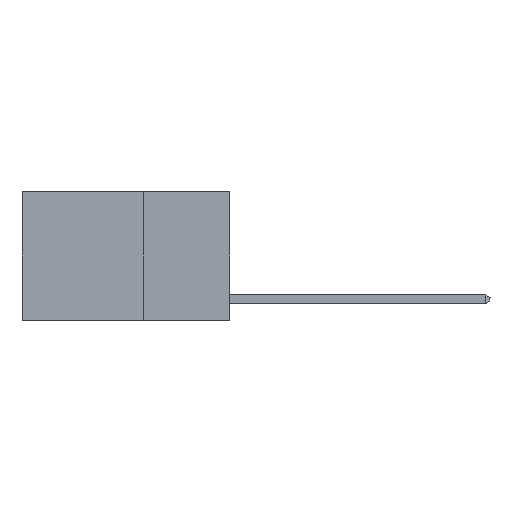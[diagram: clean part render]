
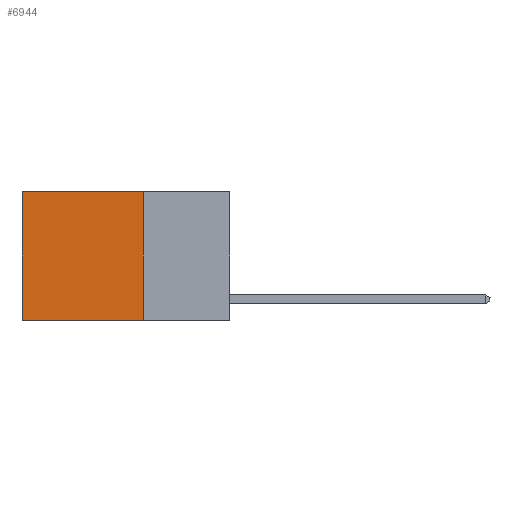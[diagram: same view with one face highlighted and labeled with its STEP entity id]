
A CAD part, left-side view. The second image highlights one B-rep face of the part: STEP entity #6944.
In plain terms, the highlighted planar face has unit normal (-1, 0, 0).
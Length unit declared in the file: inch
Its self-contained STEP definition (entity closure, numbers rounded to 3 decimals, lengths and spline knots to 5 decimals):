
#1511 = CARTESIAN_POINT ( 'NONE',  ( 0.2625, 0.6, 0. ) ) ;
#2261 = DIRECTION ( 'NONE',  ( 0., 1., 0. ) ) ;
#2919 = VERTEX_POINT ( 'NONE', #18319 ) ;
#5764 = FACE_OUTER_BOUND ( 'NONE', #28611, .T. ) ;
#5936 = DIRECTION ( 'NONE',  ( 0., 0., -1. ) ) ;
#6759 = CARTESIAN_POINT ( 'NONE',  ( 0.2625, 0.6, -0.37 ) ) ;
#6944 = ADVANCED_FACE ( 'NONE', ( #5764 ), #14652, .F. ) ;
#8259 = EDGE_CURVE ( 'NONE', #2919, #14107, #26554, .T. ) ;
#9072 = VECTOR ( 'NONE', #15475, 39.37008 ) ;
#10255 = CARTESIAN_POINT ( 'NONE',  ( 0.2625, 0.25, 0. ) ) ;
#11265 = DIRECTION ( 'NONE',  ( 0., 0., -1. ) ) ;
#11335 = EDGE_CURVE ( 'NONE', #18884, #13769, #28578, .T. ) ;
#11547 = LINE ( 'NONE', #20720, #16125 ) ;
#13413 = CARTESIAN_POINT ( 'NONE',  ( 0.2625, 0.25, 0. ) ) ;
#13769 = VERTEX_POINT ( 'NONE', #1511 ) ;
#14107 = VERTEX_POINT ( 'NONE', #6759 ) ;
#14470 = AXIS2_PLACEMENT_3D ( 'NONE', #10255, #21464, #21610 ) ;
#14652 = PLANE ( 'NONE',  #14470 ) ;
#14909 = ORIENTED_EDGE ( 'NONE', *, *, #26028, .T. ) ;
#15475 = DIRECTION ( 'NONE',  ( 0., 1., 0. ) ) ;
#15933 = VECTOR ( 'NONE', #2261, 39.37008 ) ;
#16125 = VECTOR ( 'NONE', #11265, 39.37008 ) ;
#17739 = ORIENTED_EDGE ( 'NONE', *, *, #8259, .F. ) ;
#18319 = CARTESIAN_POINT ( 'NONE',  ( 0.2625, 0.25, -0.37 ) ) ;
#18644 = VECTOR ( 'NONE', #5936, 39.37008 ) ;
#18884 = VERTEX_POINT ( 'NONE', #21972 ) ;
#19446 = EDGE_CURVE ( 'NONE', #18884, #2919, #11547, .T. ) ;
#19841 = CARTESIAN_POINT ( 'NONE',  ( 0.2625, 0.25, -0.37 ) ) ;
#20720 = CARTESIAN_POINT ( 'NONE',  ( 0.2625, 0.25, 0. ) ) ;
#21464 = DIRECTION ( 'NONE',  ( 1., 0., 0. ) ) ;
#21610 = DIRECTION ( 'NONE',  ( 0., 0., -1. ) ) ;
#21972 = CARTESIAN_POINT ( 'NONE',  ( 0.2625, 0.25, 0. ) ) ;
#23614 = ORIENTED_EDGE ( 'NONE', *, *, #11335, .T. ) ;
#25029 = ORIENTED_EDGE ( 'NONE', *, *, #19446, .F. ) ;
#25879 = CARTESIAN_POINT ( 'NONE',  ( 0.2625, 0.6, 0. ) ) ;
#26028 = EDGE_CURVE ( 'NONE', #13769, #14107, #28078, .T. ) ;
#26554 = LINE ( 'NONE', #19841, #15933 ) ;
#28078 = LINE ( 'NONE', #25879, #18644 ) ;
#28578 = LINE ( 'NONE', #13413, #9072 ) ;
#28611 = EDGE_LOOP ( 'NONE', ( #14909, #17739, #25029, #23614 ) ) ;
